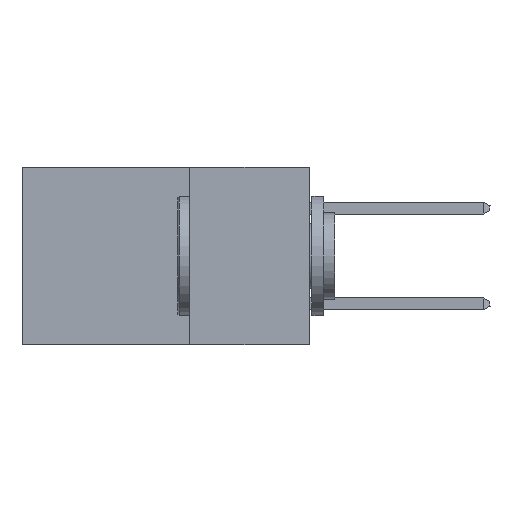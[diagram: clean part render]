
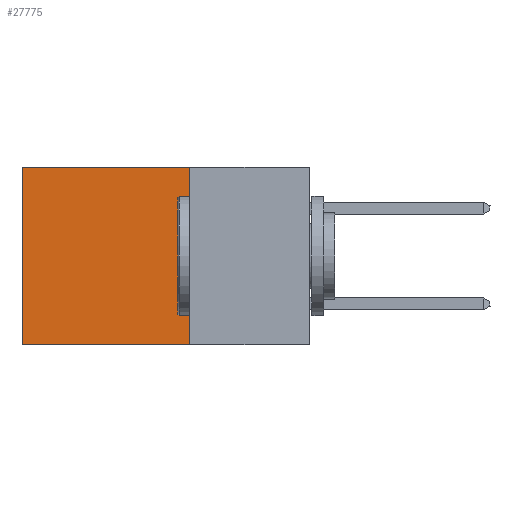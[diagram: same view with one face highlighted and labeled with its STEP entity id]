
A CAD part, left-side view. The second image highlights one B-rep face of the part: STEP entity #27775.
In plain terms, the highlighted planar face has unit normal (-1, 0, 0).
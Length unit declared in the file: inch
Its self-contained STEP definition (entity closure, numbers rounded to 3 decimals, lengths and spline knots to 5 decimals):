
#245 = EDGE_CURVE ( 'NONE', #13429, #28224, #36921, .T. ) ;
#987 = CARTESIAN_POINT ( 'NONE',  ( 0.2875, 0.25, 0. ) ) ;
#1141 = LINE ( 'NONE', #6549, #32368 ) ;
#2841 = AXIS2_PLACEMENT_3D ( 'NONE', #987, #4227, #26205 ) ;
#3410 = ORIENTED_EDGE ( 'NONE', *, *, #22499, .T. ) ;
#3606 = DIRECTION ( 'NONE',  ( 0., 1., 0. ) ) ;
#4227 = DIRECTION ( 'NONE',  ( 1., 0., 0. ) ) ;
#6549 = CARTESIAN_POINT ( 'NONE',  ( 0.2875, 0.25, -0.37 ) ) ;
#13429 = VERTEX_POINT ( 'NONE', #31121 ) ;
#16938 = CARTESIAN_POINT ( 'NONE',  ( 0.2875, 0.6, 0. ) ) ;
#18088 = ORIENTED_EDGE ( 'NONE', *, *, #245, .F. ) ;
#18984 = CARTESIAN_POINT ( 'NONE',  ( 0.2875, 0.25, 0. ) ) ;
#19015 = ORIENTED_EDGE ( 'NONE', *, *, #24414, .F. ) ;
#19507 = VERTEX_POINT ( 'NONE', #33198 ) ;
#19643 = CARTESIAN_POINT ( 'NONE',  ( 0.2875, 0.25, -0.37 ) ) ;
#22124 = VERTEX_POINT ( 'NONE', #16938 ) ;
#22182 = VECTOR ( 'NONE', #33776, 39.37008 ) ;
#22307 = DIRECTION ( 'NONE',  ( 0., 1., 0. ) ) ;
#22499 = EDGE_CURVE ( 'NONE', #22124, #19507, #30191, .T. ) ;
#22682 = EDGE_CURVE ( 'NONE', #13429, #22124, #32517, .T. ) ;
#24130 = ORIENTED_EDGE ( 'NONE', *, *, #22682, .T. ) ;
#24414 = EDGE_CURVE ( 'NONE', #28224, #19507, #1141, .T. ) ;
#24843 = DIRECTION ( 'NONE',  ( 0., 0., -1. ) ) ;
#26205 = DIRECTION ( 'NONE',  ( 0., 0., -1. ) ) ;
#26272 = EDGE_LOOP ( 'NONE', ( #3410, #19015, #18088, #24130 ) ) ;
#27775 = ADVANCED_FACE ( 'NONE', ( #33833 ), #38130, .F. ) ;
#28224 = VERTEX_POINT ( 'NONE', #19643 ) ;
#28937 = VECTOR ( 'NONE', #24843, 39.37008 ) ;
#30191 = LINE ( 'NONE', #30742, #22182 ) ;
#30643 = VECTOR ( 'NONE', #3606, 39.37008 ) ;
#30742 = CARTESIAN_POINT ( 'NONE',  ( 0.2875, 0.6, 0. ) ) ;
#31121 = CARTESIAN_POINT ( 'NONE',  ( 0.2875, 0.25, 0. ) ) ;
#32368 = VECTOR ( 'NONE', #22307, 39.37008 ) ;
#32517 = LINE ( 'NONE', #37553, #30643 ) ;
#33198 = CARTESIAN_POINT ( 'NONE',  ( 0.2875, 0.6, -0.37 ) ) ;
#33776 = DIRECTION ( 'NONE',  ( 0., 0., -1. ) ) ;
#33833 = FACE_OUTER_BOUND ( 'NONE', #26272, .T. ) ;
#36921 = LINE ( 'NONE', #18984, #28937 ) ;
#37553 = CARTESIAN_POINT ( 'NONE',  ( 0.2875, 0.25, 0. ) ) ;
#38130 = PLANE ( 'NONE',  #2841 ) ;
